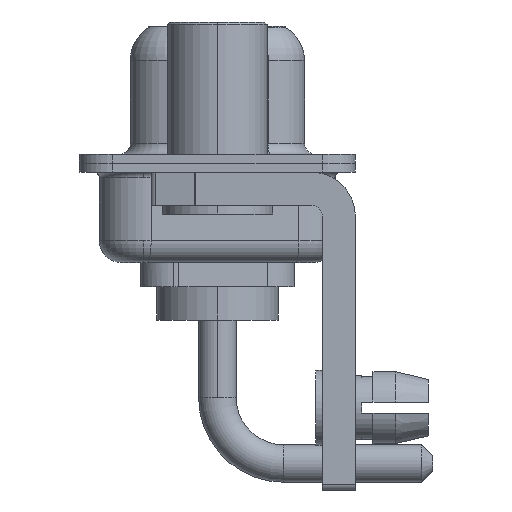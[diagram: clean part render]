
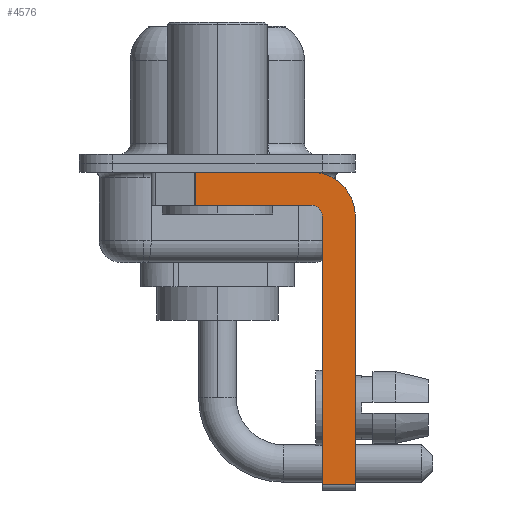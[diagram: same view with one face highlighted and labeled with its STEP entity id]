
A CAD part, left-side view. The second image highlights one B-rep face of the part: STEP entity #4576.
In plain terms, the highlighted planar face has unit normal (-1, 0, 0).
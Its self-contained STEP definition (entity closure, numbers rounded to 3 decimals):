
#1022 = VECTOR ( 'NONE', #7272, 1000. ) ;
#1142 = EDGE_CURVE ( 'NONE', #6255, #9939, #10613, .T. ) ;
#1392 = CARTESIAN_POINT ( 'NONE',  ( -2.9, 0.978, -0.4 ) ) ;
#2191 = PLANE ( 'NONE',  #6231 ) ;
#2208 = LINE ( 'NONE', #6263, #9148 ) ;
#2321 = LINE ( 'NONE', #2493, #15246 ) ;
#2493 = CARTESIAN_POINT ( 'NONE',  ( -2.9, -4.25, -1.9 ) ) ;
#3166 = EDGE_CURVE ( 'NONE', #13823, #4708, #7464, .T. ) ;
#3284 = EDGE_CURVE ( 'NONE', #9803, #10098, #13553, .T. ) ;
#3450 = ORIENTED_EDGE ( 'NONE', *, *, #3166, .F. ) ;
#3454 = EDGE_CURVE ( 'NONE', #6255, #13823, #6110, .T. ) ;
#3852 = CARTESIAN_POINT ( 'NONE',  ( -2.9, -4.25, -2.4 ) ) ;
#4576 = ADVANCED_FACE ( 'NONE', ( #8831 ), #2191, .F. ) ;
#4708 = VERTEX_POINT ( 'NONE', #7934 ) ;
#4921 = AXIS2_PLACEMENT_3D ( 'NONE', #13997, #7360, #11189 ) ;
#4940 = DIRECTION ( 'NONE',  ( 0., 0., 1. ) ) ;
#5089 = DIRECTION ( 'NONE',  ( 1., 0., 0. ) ) ;
#5489 = DIRECTION ( 'NONE',  ( 0., 0., -1. ) ) ;
#5922 = ORIENTED_EDGE ( 'NONE', *, *, #8844, .F. ) ;
#5941 = ORIENTED_EDGE ( 'NONE', *, *, #3284, .T. ) ;
#5998 = VERTEX_POINT ( 'NONE', #15174 ) ;
#6110 = LINE ( 'NONE', #15223, #1022 ) ;
#6231 = AXIS2_PLACEMENT_3D ( 'NONE', #6421, #5089, #15878 ) ;
#6255 = VERTEX_POINT ( 'NONE', #1392 ) ;
#6263 = CARTESIAN_POINT ( 'NONE',  ( -2.9, -4.75, -14.8 ) ) ;
#6421 = CARTESIAN_POINT ( 'NONE',  ( -2.9, -4.25, -2.4 ) ) ;
#6477 = DIRECTION ( 'NONE',  ( 0., 0., -1. ) ) ;
#7272 = DIRECTION ( 'NONE',  ( 0., -1., 0. ) ) ;
#7360 = DIRECTION ( 'NONE',  ( -1., 0., 0. ) ) ;
#7464 = CIRCLE ( 'NONE', #10008, 2. ) ;
#7538 = CARTESIAN_POINT ( 'NONE',  ( -2.9, -4.25, -1.9 ) ) ;
#7876 = DIRECTION ( 'NONE',  ( 0., 1., 0. ) ) ;
#7934 = CARTESIAN_POINT ( 'NONE',  ( -2.9, -6.25, -2.4 ) ) ;
#8831 = FACE_OUTER_BOUND ( 'NONE', #16451, .T. ) ;
#8844 = EDGE_CURVE ( 'NONE', #4708, #10098, #15852, .T. ) ;
#8980 = ORIENTED_EDGE ( 'NONE', *, *, #1142, .T. ) ;
#9090 = CARTESIAN_POINT ( 'NONE',  ( -2.9, -4.75, -14.55 ) ) ;
#9148 = VECTOR ( 'NONE', #4940, 1000. ) ;
#9803 = VERTEX_POINT ( 'NONE', #9090 ) ;
#9899 = ORIENTED_EDGE ( 'NONE', *, *, #10190, .F. ) ;
#9939 = VERTEX_POINT ( 'NONE', #14732 ) ;
#10008 = AXIS2_PLACEMENT_3D ( 'NONE', #3852, #15850, #6477 ) ;
#10098 = VERTEX_POINT ( 'NONE', #10343 ) ;
#10190 = EDGE_CURVE ( 'NONE', #9803, #5998, #2208, .T. ) ;
#10310 = CARTESIAN_POINT ( 'NONE',  ( -2.9, -6.25, -2.4 ) ) ;
#10343 = CARTESIAN_POINT ( 'NONE',  ( -2.9, -6.25, -14.55 ) ) ;
#10377 = VERTEX_POINT ( 'NONE', #7538 ) ;
#10459 = ORIENTED_EDGE ( 'NONE', *, *, #13222, .F. ) ;
#10613 = LINE ( 'NONE', #15991, #10707 ) ;
#10707 = VECTOR ( 'NONE', #5489, 1000. ) ;
#11005 = CARTESIAN_POINT ( 'NONE',  ( -2.9, -4.25, -14.55 ) ) ;
#11137 = EDGE_CURVE ( 'NONE', #5998, #10377, #11163, .T. ) ;
#11163 = CIRCLE ( 'NONE', #4921, 0.5 ) ;
#11189 = DIRECTION ( 'NONE',  ( 0., 0., 1. ) ) ;
#11449 = CARTESIAN_POINT ( 'NONE',  ( -2.9, -4.25, -0.4 ) ) ;
#12933 = DIRECTION ( 'NONE',  ( 0., 0., -1. ) ) ;
#13222 = EDGE_CURVE ( 'NONE', #10377, #9939, #2321, .T. ) ;
#13553 = LINE ( 'NONE', #11005, #15893 ) ;
#13781 = ORIENTED_EDGE ( 'NONE', *, *, #3454, .F. ) ;
#13823 = VERTEX_POINT ( 'NONE', #11449 ) ;
#13910 = VECTOR ( 'NONE', #12933, 1000. ) ;
#13997 = CARTESIAN_POINT ( 'NONE',  ( -2.9, -4.25, -2.4 ) ) ;
#14732 = CARTESIAN_POINT ( 'NONE',  ( -2.9, 0.978, -1.9 ) ) ;
#15174 = CARTESIAN_POINT ( 'NONE',  ( -2.9, -4.75, -2.4 ) ) ;
#15223 = CARTESIAN_POINT ( 'NONE',  ( -2.9, 3., -0.4 ) ) ;
#15246 = VECTOR ( 'NONE', #7876, 1000. ) ;
#15850 = DIRECTION ( 'NONE',  ( 1., 0., 0. ) ) ;
#15852 = LINE ( 'NONE', #10310, #13910 ) ;
#15878 = DIRECTION ( 'NONE',  ( 0., 0., -1. ) ) ;
#15893 = VECTOR ( 'NONE', #16122, 1000. ) ;
#15991 = CARTESIAN_POINT ( 'NONE',  ( -2.9, 0.978, -1.9 ) ) ;
#16122 = DIRECTION ( 'NONE',  ( 0., -1., 0. ) ) ;
#16451 = EDGE_LOOP ( 'NONE', ( #13781, #8980, #10459, #17194, #9899, #5941, #5922, #3450 ) ) ;
#17194 = ORIENTED_EDGE ( 'NONE', *, *, #11137, .F. ) ;
